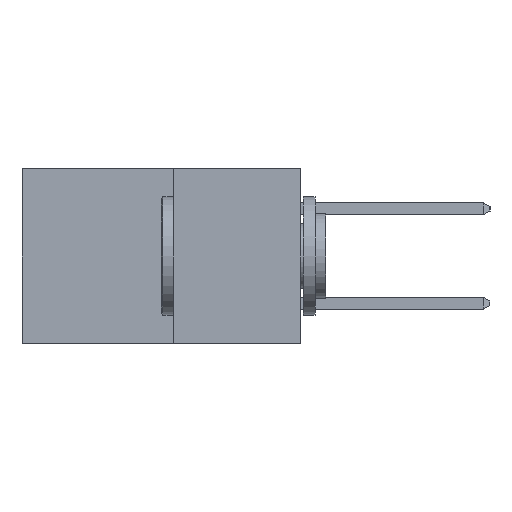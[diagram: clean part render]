
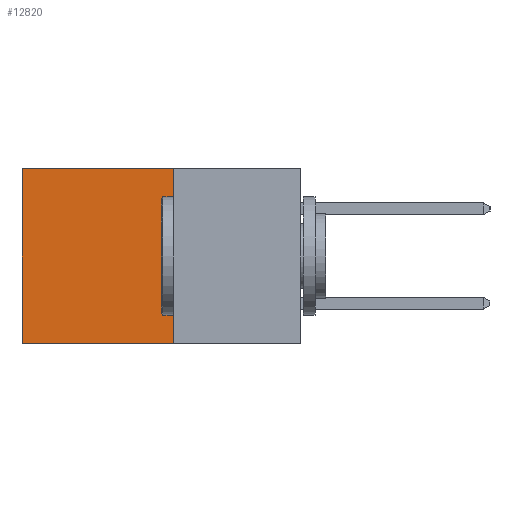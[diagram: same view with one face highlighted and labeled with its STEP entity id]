
A CAD part, left-side view. The second image highlights one B-rep face of the part: STEP entity #12820.
In plain terms, the highlighted planar face has unit normal (-1, 0, 0).
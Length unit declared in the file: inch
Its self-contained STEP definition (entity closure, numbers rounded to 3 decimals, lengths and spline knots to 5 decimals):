
#419 = VECTOR ( 'NONE', #9003, 39.37008 ) ;
#874 = VERTEX_POINT ( 'NONE', #13010 ) ;
#1529 = VECTOR ( 'NONE', #10094, 39.37008 ) ;
#1542 = LINE ( 'NONE', #4609, #8068 ) ;
#1651 = CARTESIAN_POINT ( 'NONE',  ( 0.277, 0.59, -0.37 ) ) ;
#2395 = ORIENTED_EDGE ( 'NONE', *, *, #9795, .T. ) ;
#2411 = CARTESIAN_POINT ( 'NONE',  ( 0.277, 0.27, 0. ) ) ;
#2568 = DIRECTION ( 'NONE',  ( 1., 0., 0. ) ) ;
#3455 = FACE_OUTER_BOUND ( 'NONE', #10727, .T. ) ;
#4181 = EDGE_CURVE ( 'NONE', #13449, #9094, #1542, .T. ) ;
#4609 = CARTESIAN_POINT ( 'NONE',  ( 0.277, 0.27, -0.37 ) ) ;
#7697 = DIRECTION ( 'NONE',  ( 0., 0., -1. ) ) ;
#8068 = VECTOR ( 'NONE', #7697, 39.37008 ) ;
#8485 = DIRECTION ( 'NONE',  ( 0., 0., -1. ) ) ;
#8724 = EDGE_CURVE ( 'NONE', #9094, #874, #11499, .T. ) ;
#8883 = LINE ( 'NONE', #12845, #1529 ) ;
#9003 = DIRECTION ( 'NONE',  ( 0., 1., 0. ) ) ;
#9094 = VERTEX_POINT ( 'NONE', #15508 ) ;
#9284 = CARTESIAN_POINT ( 'NONE',  ( 0.277, 0.27, -0.37 ) ) ;
#9688 = EDGE_CURVE ( 'NONE', #12074, #874, #13837, .T. ) ;
#9795 = EDGE_CURVE ( 'NONE', #13449, #12074, #8883, .T. ) ;
#10094 = DIRECTION ( 'NONE',  ( 0., 1., 0. ) ) ;
#10596 = VECTOR ( 'NONE', #8485, 39.37008 ) ;
#10727 = EDGE_LOOP ( 'NONE', ( #13774, #13998, #16091, #2395 ) ) ;
#10768 = CARTESIAN_POINT ( 'NONE',  ( 0.277, 0.27, -0.37 ) ) ;
#11499 = LINE ( 'NONE', #9284, #419 ) ;
#12074 = VERTEX_POINT ( 'NONE', #12105 ) ;
#12105 = CARTESIAN_POINT ( 'NONE',  ( 0.277, 0.59, 0. ) ) ;
#12183 = DIRECTION ( 'NONE',  ( 0., 0., -1. ) ) ;
#12820 = ADVANCED_FACE ( 'NONE', ( #3455 ), #13502, .F. ) ;
#12845 = CARTESIAN_POINT ( 'NONE',  ( 0.277, 0.27, 0. ) ) ;
#13010 = CARTESIAN_POINT ( 'NONE',  ( 0.277, 0.59, -0.37 ) ) ;
#13449 = VERTEX_POINT ( 'NONE', #2411 ) ;
#13502 = PLANE ( 'NONE',  #13975 ) ;
#13774 = ORIENTED_EDGE ( 'NONE', *, *, #9688, .T. ) ;
#13837 = LINE ( 'NONE', #1651, #10596 ) ;
#13975 = AXIS2_PLACEMENT_3D ( 'NONE', #10768, #2568, #12183 ) ;
#13998 = ORIENTED_EDGE ( 'NONE', *, *, #8724, .F. ) ;
#15508 = CARTESIAN_POINT ( 'NONE',  ( 0.277, 0.27, -0.37 ) ) ;
#16091 = ORIENTED_EDGE ( 'NONE', *, *, #4181, .F. ) ;
